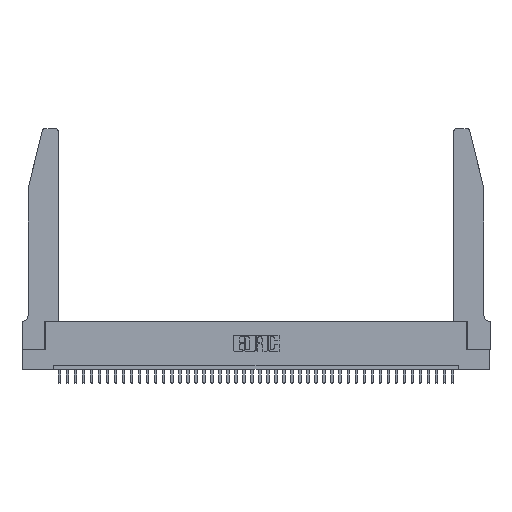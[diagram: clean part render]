
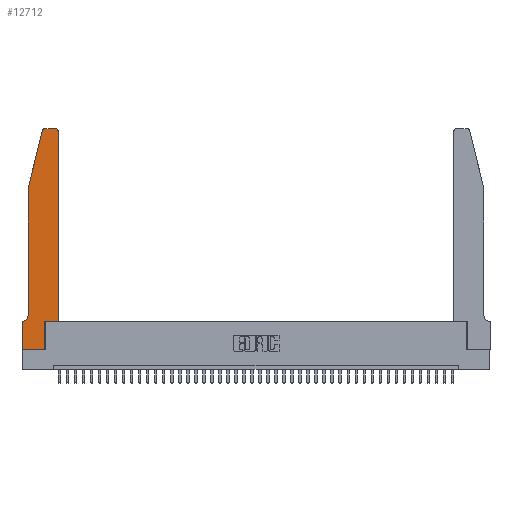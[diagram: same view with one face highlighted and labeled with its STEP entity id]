
A CAD part, top view. The second image highlights one B-rep face of the part: STEP entity #12712.
In plain terms, the highlighted planar face has unit normal (0, 0, 1).
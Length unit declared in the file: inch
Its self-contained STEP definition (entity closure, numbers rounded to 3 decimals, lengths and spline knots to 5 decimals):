
#114 = EDGE_CURVE ( 'NONE', #7701, #23471, #37380, .T. ) ;
#256 = VERTEX_POINT ( 'NONE', #3723 ) ;
#831 = DIRECTION ( 'NONE',  ( 0., 0., 1. ) ) ;
#976 = CARTESIAN_POINT ( 'NONE',  ( 0.2605, 2.75, 0.37 ) ) ;
#1323 = VERTEX_POINT ( 'NONE', #2801 ) ;
#1519 = CARTESIAN_POINT ( 'NONE',  ( 0.2865, 0.35, 0.37 ) ) ;
#2030 = CARTESIAN_POINT ( 'NONE',  ( 0.4505, 0.35, 0.37 ) ) ;
#2317 = EDGE_CURVE ( 'NONE', #32680, #31774, #16706, .T. ) ;
#2658 = VECTOR ( 'NONE', #17327, 39.37008 ) ;
#2710 = AXIS2_PLACEMENT_3D ( 'NONE', #29282, #10129, #16585 ) ;
#2773 = CARTESIAN_POINT ( 'NONE',  ( 0.4205, 2.75, 0.37 ) ) ;
#2801 = CARTESIAN_POINT ( 'NONE',  ( 0.0055, 0.35, 0.37 ) ) ;
#3263 = CARTESIAN_POINT ( 'NONE',  ( 0.25487, 2.72718, 0.37 ) ) ;
#3628 = CIRCLE ( 'NONE', #35156, 0.03 ) ;
#3718 = EDGE_CURVE ( 'NONE', #15950, #256, #30094, .T. ) ;
#3723 = CARTESIAN_POINT ( 'NONE',  ( 0.4505, 2.72, 0.37 ) ) ;
#4067 = DIRECTION ( 'NONE',  ( 1., 0., 0. ) ) ;
#4120 = ORIENTED_EDGE ( 'NONE', *, *, #16126, .T. ) ;
#4862 = CARTESIAN_POINT ( 'NONE',  ( 0.2865, 0.35, 0.37 ) ) ;
#5424 = VECTOR ( 'NONE', #36919, 39.37008 ) ;
#6005 = VECTOR ( 'NONE', #8974, 39.37008 ) ;
#6787 = FACE_OUTER_BOUND ( 'NONE', #19099, .T. ) ;
#6814 = VECTOR ( 'NONE', #13867, 39.37008 ) ;
#7582 = DIRECTION ( 'NONE',  ( 0., 0., 1. ) ) ;
#7701 = VERTEX_POINT ( 'NONE', #8053 ) ;
#8014 = ORIENTED_EDGE ( 'NONE', *, *, #24867, .T. ) ;
#8053 = CARTESIAN_POINT ( 'NONE',  ( 0., 0., 0.37 ) ) ;
#8726 = DIRECTION ( 'NONE',  ( -0.239, -0.971, 0. ) ) ;
#8761 = CARTESIAN_POINT ( 'NONE',  ( 0.2865, 0., 0.37 ) ) ;
#8974 = DIRECTION ( 'NONE',  ( 0., -1., 0. ) ) ;
#9127 = VECTOR ( 'NONE', #29033, 39.37008 ) ;
#10129 = DIRECTION ( 'NONE',  ( 0., 0., -1. ) ) ;
#10214 = CARTESIAN_POINT ( 'NONE',  ( 0.0755, 2., 0.37 ) ) ;
#10219 = ORIENTED_EDGE ( 'NONE', *, *, #14072, .T. ) ;
#10490 = EDGE_CURVE ( 'NONE', #40426, #15950, #12261, .T. ) ;
#11538 = EDGE_CURVE ( 'NONE', #16234, #12635, #16920, .T. ) ;
#11663 = DIRECTION ( 'NONE',  ( 1., 0., 0. ) ) ;
#12261 = LINE ( 'NONE', #37805, #29099 ) ;
#12452 = VECTOR ( 'NONE', #13848, 39.37008 ) ;
#12635 = VERTEX_POINT ( 'NONE', #21556 ) ;
#12712 = ADVANCED_FACE ( 'NONE', ( #6787 ), #24515, .T. ) ;
#12965 = VECTOR ( 'NONE', #8726, 39.37008 ) ;
#13848 = DIRECTION ( 'NONE',  ( -1., 0., 0. ) ) ;
#13867 = DIRECTION ( 'NONE',  ( 1., 0., 0. ) ) ;
#14019 = DIRECTION ( 'NONE',  ( 1., 0., 0. ) ) ;
#14072 = EDGE_CURVE ( 'NONE', #12635, #40735, #3628, .T. ) ;
#14811 = EDGE_CURVE ( 'NONE', #256, #16234, #16139, .T. ) ;
#14853 = VERTEX_POINT ( 'NONE', #16977 ) ;
#15372 = AXIS2_PLACEMENT_3D ( 'NONE', #33016, #831, #4067 ) ;
#15950 = VERTEX_POINT ( 'NONE', #30428 ) ;
#16126 = EDGE_CURVE ( 'NONE', #14853, #7701, #31985, .T. ) ;
#16139 = CIRCLE ( 'NONE', #15372, 0.03 ) ;
#16234 = VERTEX_POINT ( 'NONE', #2773 ) ;
#16585 = DIRECTION ( 'NONE',  ( -1., 0., 0. ) ) ;
#16706 = LINE ( 'NONE', #10214, #39182 ) ;
#16920 = LINE ( 'NONE', #976, #12452 ) ;
#16977 = CARTESIAN_POINT ( 'NONE',  ( 0., 0.35, 0.37 ) ) ;
#17009 = EDGE_CURVE ( 'NONE', #31774, #1323, #25271, .T. ) ;
#17020 = ORIENTED_EDGE ( 'NONE', *, *, #14811, .T. ) ;
#17327 = DIRECTION ( 'NONE',  ( -1., 0., 0. ) ) ;
#18669 = DIRECTION ( 'NONE',  ( 1., 0., 0. ) ) ;
#19099 = EDGE_LOOP ( 'NONE', ( #22490, #10219, #34768, #39599, #34695, #8014, #4120, #28562, #30383, #33399, #34993, #17020 ) ) ;
#19919 = EDGE_CURVE ( 'NONE', #40735, #32680, #31508, .T. ) ;
#20697 = CARTESIAN_POINT ( 'NONE',  ( 0., 0., 0.37 ) ) ;
#21556 = CARTESIAN_POINT ( 'NONE',  ( 0.284, 2.75, 0.37 ) ) ;
#22047 = CARTESIAN_POINT ( 'NONE',  ( 0.0755, 0.42, 0.37 ) ) ;
#22490 = ORIENTED_EDGE ( 'NONE', *, *, #11538, .T. ) ;
#23035 = DIRECTION ( 'NONE',  ( 0., -1., 0. ) ) ;
#23343 = LINE ( 'NONE', #1519, #5424 ) ;
#23471 = VERTEX_POINT ( 'NONE', #8761 ) ;
#24515 = PLANE ( 'NONE',  #32665 ) ;
#24867 = EDGE_CURVE ( 'NONE', #1323, #14853, #29113, .T. ) ;
#25202 = CARTESIAN_POINT ( 'NONE',  ( 0.0755, 2., 0.37 ) ) ;
#25271 = CIRCLE ( 'NONE', #2710, 0.07 ) ;
#26514 = CARTESIAN_POINT ( 'NONE',  ( 0.0755, 0.35, 0.37 ) ) ;
#26706 = CARTESIAN_POINT ( 'NONE',  ( 0.284, 2.72, 0.37 ) ) ;
#28252 = CARTESIAN_POINT ( 'NONE',  ( 0., 0.35, 0.37 ) ) ;
#28562 = ORIENTED_EDGE ( 'NONE', *, *, #114, .T. ) ;
#29033 = DIRECTION ( 'NONE',  ( 0., 1., 0. ) ) ;
#29099 = VECTOR ( 'NONE', #18669, 39.37008 ) ;
#29113 = LINE ( 'NONE', #26514, #2658 ) ;
#29282 = CARTESIAN_POINT ( 'NONE',  ( 0.0055, 0.42, 0.37 ) ) ;
#30094 = LINE ( 'NONE', #2030, #9127 ) ;
#30383 = ORIENTED_EDGE ( 'NONE', *, *, #31535, .T. ) ;
#30428 = CARTESIAN_POINT ( 'NONE',  ( 0.4505, 0.35, 0.37 ) ) ;
#30784 = DIRECTION ( 'NONE',  ( 0., 0., 1. ) ) ;
#30923 = CARTESIAN_POINT ( 'NONE',  ( 0.0755, 2., 0.37 ) ) ;
#31508 = LINE ( 'NONE', #30923, #12965 ) ;
#31535 = EDGE_CURVE ( 'NONE', #23471, #40426, #23343, .T. ) ;
#31774 = VERTEX_POINT ( 'NONE', #22047 ) ;
#31985 = LINE ( 'NONE', #40582, #6005 ) ;
#32665 = AXIS2_PLACEMENT_3D ( 'NONE', #28252, #30784, #11663 ) ;
#32680 = VERTEX_POINT ( 'NONE', #25202 ) ;
#33016 = CARTESIAN_POINT ( 'NONE',  ( 0.4205, 2.72, 0.37 ) ) ;
#33399 = ORIENTED_EDGE ( 'NONE', *, *, #10490, .T. ) ;
#34695 = ORIENTED_EDGE ( 'NONE', *, *, #17009, .T. ) ;
#34768 = ORIENTED_EDGE ( 'NONE', *, *, #19919, .T. ) ;
#34993 = ORIENTED_EDGE ( 'NONE', *, *, #3718, .T. ) ;
#35156 = AXIS2_PLACEMENT_3D ( 'NONE', #26706, #7582, #14019 ) ;
#36919 = DIRECTION ( 'NONE',  ( 0., 1., 0. ) ) ;
#37380 = LINE ( 'NONE', #20697, #6814 ) ;
#37805 = CARTESIAN_POINT ( 'NONE',  ( 0.4505, 0.35, 0.37 ) ) ;
#39182 = VECTOR ( 'NONE', #23035, 39.37008 ) ;
#39599 = ORIENTED_EDGE ( 'NONE', *, *, #2317, .T. ) ;
#40426 = VERTEX_POINT ( 'NONE', #4862 ) ;
#40582 = CARTESIAN_POINT ( 'NONE',  ( 0., 0., 0.37 ) ) ;
#40735 = VERTEX_POINT ( 'NONE', #3263 ) ;
